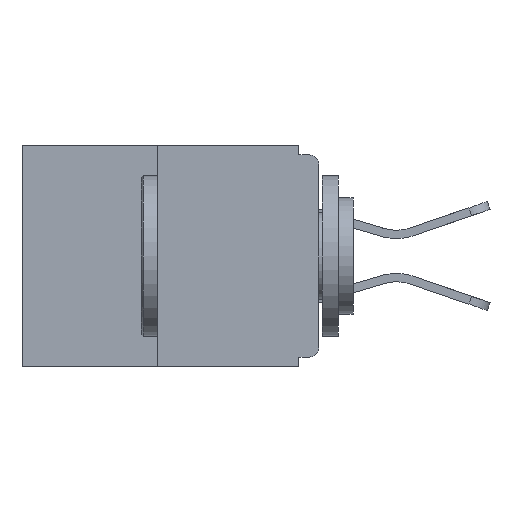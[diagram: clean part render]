
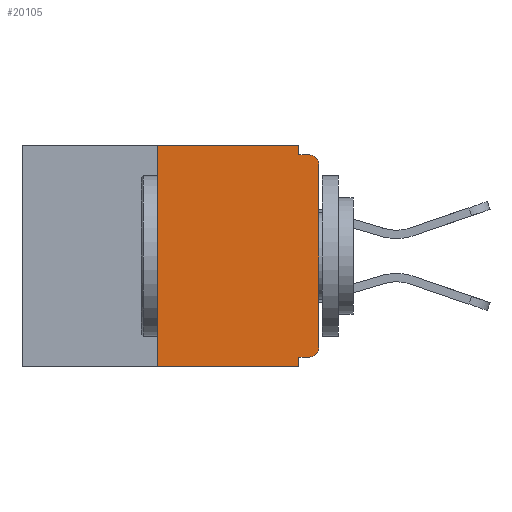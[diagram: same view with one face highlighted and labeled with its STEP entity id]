
A CAD part, left-side view. The second image highlights one B-rep face of the part: STEP entity #20105.
In plain terms, the highlighted planar face has unit normal (-1, 0, 0).
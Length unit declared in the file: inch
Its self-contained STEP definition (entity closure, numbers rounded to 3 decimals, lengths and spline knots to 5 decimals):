
#145 = CARTESIAN_POINT ( 'NONE',  ( 0., 0.015, -0.328 ) ) ;
#540 = CARTESIAN_POINT ( 'NONE',  ( 0., 0., -0.015 ) ) ;
#824 = EDGE_CURVE ( 'NONE', #5616, #13645, #12338, .T. ) ;
#1129 = DIRECTION ( 'NONE',  ( -1., 0., 0. ) ) ;
#1186 = CARTESIAN_POINT ( 'NONE',  ( 0., 0.015, -0.313 ) ) ;
#1398 = LINE ( 'NONE', #25901, #9242 ) ;
#2136 = CARTESIAN_POINT ( 'NONE',  ( 0., 0., 0. ) ) ;
#2503 = ORIENTED_EDGE ( 'NONE', *, *, #15033, .F. ) ;
#2574 = CARTESIAN_POINT ( 'NONE',  ( 0., 0.25, 0. ) ) ;
#2962 = ORIENTED_EDGE ( 'NONE', *, *, #24170, .F. ) ;
#3038 = DIRECTION ( 'NONE',  ( 0., -1., 0. ) ) ;
#3294 = PLANE ( 'NONE',  #6212 ) ;
#3331 = EDGE_CURVE ( 'NONE', #7137, #19189, #1398, .T. ) ;
#4544 = EDGE_CURVE ( 'NONE', #5075, #22735, #14515, .T. ) ;
#4856 = DIRECTION ( 'NONE',  ( -1., 0., 0. ) ) ;
#4921 = CARTESIAN_POINT ( 'NONE',  ( 0., 0., -0.328 ) ) ;
#5075 = VERTEX_POINT ( 'NONE', #21755 ) ;
#5148 = CARTESIAN_POINT ( 'NONE',  ( 0., 0.46, 0. ) ) ;
#5433 = VERTEX_POINT ( 'NONE', #5784 ) ;
#5504 = DIRECTION ( 'NONE',  ( 0., 0., -1. ) ) ;
#5576 = VECTOR ( 'NONE', #24320, 39.37008 ) ;
#5616 = VERTEX_POINT ( 'NONE', #145 ) ;
#5635 = LINE ( 'NONE', #540, #20637 ) ;
#5784 = CARTESIAN_POINT ( 'NONE',  ( 0., 0., -0.03 ) ) ;
#5901 = DIRECTION ( 'NONE',  ( 0., 0., 1. ) ) ;
#6212 = AXIS2_PLACEMENT_3D ( 'NONE', #9357, #15425, #5504 ) ;
#6255 = ORIENTED_EDGE ( 'NONE', *, *, #824, .T. ) ;
#6782 = DIRECTION ( 'NONE',  ( 0., 0., -1. ) ) ;
#7137 = VERTEX_POINT ( 'NONE', #18743 ) ;
#7284 = VECTOR ( 'NONE', #12581, 39.37008 ) ;
#7756 = CARTESIAN_POINT ( 'NONE',  ( 0., 0.031, -0.015 ) ) ;
#7914 = CARTESIAN_POINT ( 'NONE',  ( 0., 0.46, -0.343 ) ) ;
#8071 = EDGE_CURVE ( 'NONE', #9917, #19189, #20265, .T. ) ;
#8092 = DIRECTION ( 'NONE',  ( 0., -1., 0. ) ) ;
#8400 = VECTOR ( 'NONE', #3038, 39.37008 ) ;
#8580 = VECTOR ( 'NONE', #8620, 39.37008 ) ;
#8620 = DIRECTION ( 'NONE',  ( 0., 0., 1. ) ) ;
#9119 = ORIENTED_EDGE ( 'NONE', *, *, #17233, .T. ) ;
#9242 = VECTOR ( 'NONE', #17992, 39.37008 ) ;
#9357 = CARTESIAN_POINT ( 'NONE',  ( 0., 0.46, 0. ) ) ;
#9917 = VERTEX_POINT ( 'NONE', #14907 ) ;
#10796 = ORIENTED_EDGE ( 'NONE', *, *, #8071, .T. ) ;
#11596 = EDGE_CURVE ( 'NONE', #15855, #5075, #21577, .T. ) ;
#11705 = VECTOR ( 'NONE', #5901, 39.37008 ) ;
#12179 = CARTESIAN_POINT ( 'NONE',  ( 0., 0.25, 0. ) ) ;
#12338 = CIRCLE ( 'NONE', #22997, 0.015 ) ;
#12581 = DIRECTION ( 'NONE',  ( 0., 0., -1. ) ) ;
#12932 = LINE ( 'NONE', #4921, #25531 ) ;
#13645 = VERTEX_POINT ( 'NONE', #25284 ) ;
#14515 = LINE ( 'NONE', #24273, #7284 ) ;
#14653 = ORIENTED_EDGE ( 'NONE', *, *, #3331, .F. ) ;
#14907 = CARTESIAN_POINT ( 'NONE',  ( 0., 0.25, -0.343 ) ) ;
#15033 = EDGE_CURVE ( 'NONE', #9917, #15855, #15209, .T. ) ;
#15209 = LINE ( 'NONE', #2574, #8580 ) ;
#15229 = ORIENTED_EDGE ( 'NONE', *, *, #22089, .F. ) ;
#15259 = DIRECTION ( 'NONE',  ( 0., 0., -1. ) ) ;
#15425 = DIRECTION ( 'NONE',  ( 1., 0., 0. ) ) ;
#15434 = CARTESIAN_POINT ( 'NONE',  ( 0., 0.015, -0.03 ) ) ;
#15855 = VERTEX_POINT ( 'NONE', #12179 ) ;
#16402 = LINE ( 'NONE', #2136, #11705 ) ;
#16463 = ORIENTED_EDGE ( 'NONE', *, *, #4544, .F. ) ;
#16571 = VERTEX_POINT ( 'NONE', #20157 ) ;
#17233 = EDGE_CURVE ( 'NONE', #5433, #16571, #25128, .T. ) ;
#17992 = DIRECTION ( 'NONE',  ( 0., 0., -1. ) ) ;
#18743 = CARTESIAN_POINT ( 'NONE',  ( 0., 0.031, -0.328 ) ) ;
#19189 = VERTEX_POINT ( 'NONE', #24646 ) ;
#20105 = ADVANCED_FACE ( 'NONE', ( #23993 ), #3294, .F. ) ;
#20157 = CARTESIAN_POINT ( 'NONE',  ( 0., 0.015, -0.015 ) ) ;
#20265 = LINE ( 'NONE', #7914, #5576 ) ;
#20637 = VECTOR ( 'NONE', #8092, 39.37008 ) ;
#20869 = EDGE_CURVE ( 'NONE', #13645, #5433, #16402, .T. ) ;
#20947 = DIRECTION ( 'NONE',  ( 0., 1., 0. ) ) ;
#21226 = EDGE_LOOP ( 'NONE', ( #21745, #2503, #10796, #14653, #15229, #6255, #25787, #9119, #2962, #16463 ) ) ;
#21577 = LINE ( 'NONE', #5148, #8400 ) ;
#21745 = ORIENTED_EDGE ( 'NONE', *, *, #11596, .F. ) ;
#21755 = CARTESIAN_POINT ( 'NONE',  ( 0., 0.031, 0. ) ) ;
#22089 = EDGE_CURVE ( 'NONE', #5616, #7137, #12932, .T. ) ;
#22735 = VERTEX_POINT ( 'NONE', #7756 ) ;
#22997 = AXIS2_PLACEMENT_3D ( 'NONE', #1186, #4856, #6782 ) ;
#23309 = AXIS2_PLACEMENT_3D ( 'NONE', #15434, #1129, #15259 ) ;
#23993 = FACE_OUTER_BOUND ( 'NONE', #21226, .T. ) ;
#24170 = EDGE_CURVE ( 'NONE', #22735, #16571, #5635, .T. ) ;
#24273 = CARTESIAN_POINT ( 'NONE',  ( 0., 0.031, 0. ) ) ;
#24320 = DIRECTION ( 'NONE',  ( 0., -1., 0. ) ) ;
#24646 = CARTESIAN_POINT ( 'NONE',  ( 0., 0.031, -0.343 ) ) ;
#25128 = CIRCLE ( 'NONE', #23309, 0.015 ) ;
#25284 = CARTESIAN_POINT ( 'NONE',  ( 0., 0., -0.313 ) ) ;
#25531 = VECTOR ( 'NONE', #20947, 39.37008 ) ;
#25787 = ORIENTED_EDGE ( 'NONE', *, *, #20869, .T. ) ;
#25901 = CARTESIAN_POINT ( 'NONE',  ( 0., 0.031, -0.343 ) ) ;
